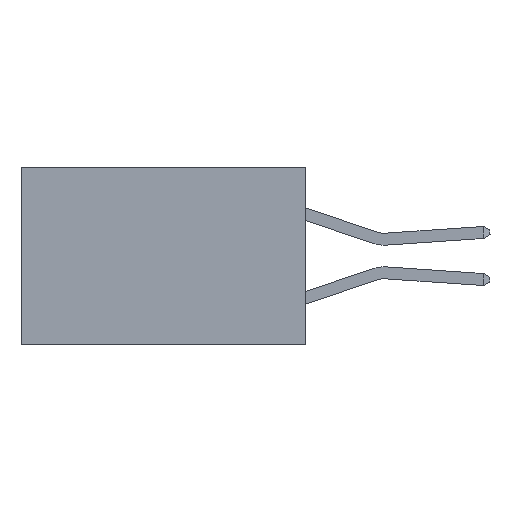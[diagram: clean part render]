
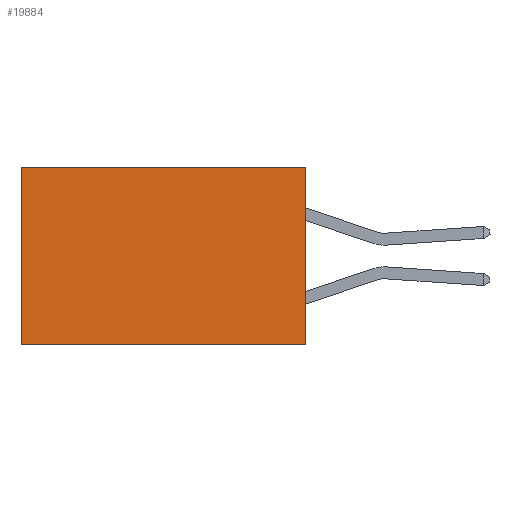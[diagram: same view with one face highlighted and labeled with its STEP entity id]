
A CAD part, left-side view. The second image highlights one B-rep face of the part: STEP entity #19884.
In plain terms, the highlighted planar face has unit normal (-1, 0, 0).
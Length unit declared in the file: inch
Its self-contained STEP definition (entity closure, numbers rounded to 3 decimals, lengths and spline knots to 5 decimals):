
#1234 = EDGE_CURVE ( 'NONE', #11306, #12728, #7090, .T. ) ;
#1339 = ORIENTED_EDGE ( 'NONE', *, *, #17410, .F. ) ;
#1686 = VECTOR ( 'NONE', #3702, 39.37008 ) ;
#2017 = DIRECTION ( 'NONE',  ( 0., 0., -1. ) ) ;
#2147 = AXIS2_PLACEMENT_3D ( 'NONE', #26123, #14279, #2017 ) ;
#3013 = CARTESIAN_POINT ( 'NONE',  ( 0.277, 0., 0. ) ) ;
#3610 = ORIENTED_EDGE ( 'NONE', *, *, #9936, .T. ) ;
#3702 = DIRECTION ( 'NONE',  ( 0., 1., 0. ) ) ;
#3708 = VERTEX_POINT ( 'NONE', #13649 ) ;
#4293 = ORIENTED_EDGE ( 'NONE', *, *, #5813, .F. ) ;
#5003 = EDGE_LOOP ( 'NONE', ( #3610, #4293, #1339, #12334 ) ) ;
#5049 = LINE ( 'NONE', #21857, #15259 ) ;
#5813 = EDGE_CURVE ( 'NONE', #3708, #24975, #5049, .T. ) ;
#6667 = LINE ( 'NONE', #12397, #22193 ) ;
#7090 = LINE ( 'NONE', #3013, #1686 ) ;
#7598 = CARTESIAN_POINT ( 'NONE',  ( 0.277, 0., -0.37 ) ) ;
#9936 = EDGE_CURVE ( 'NONE', #12728, #24975, #6667, .T. ) ;
#10819 = CARTESIAN_POINT ( 'NONE',  ( 0.277, 0.59, 0. ) ) ;
#11036 = VECTOR ( 'NONE', #11730, 39.37008 ) ;
#11306 = VERTEX_POINT ( 'NONE', #16877 ) ;
#11730 = DIRECTION ( 'NONE',  ( 0., 0., -1. ) ) ;
#12334 = ORIENTED_EDGE ( 'NONE', *, *, #1234, .T. ) ;
#12397 = CARTESIAN_POINT ( 'NONE',  ( 0.277, 0.59, -0.37 ) ) ;
#12728 = VERTEX_POINT ( 'NONE', #10819 ) ;
#13649 = CARTESIAN_POINT ( 'NONE',  ( 0.277, 0., -0.37 ) ) ;
#14279 = DIRECTION ( 'NONE',  ( 1., 0., 0. ) ) ;
#14931 = DIRECTION ( 'NONE',  ( 0., 1., 0. ) ) ;
#15259 = VECTOR ( 'NONE', #14931, 39.37008 ) ;
#16471 = LINE ( 'NONE', #7598, #11036 ) ;
#16877 = CARTESIAN_POINT ( 'NONE',  ( 0.277, 0., 0. ) ) ;
#16982 = CARTESIAN_POINT ( 'NONE',  ( 0.277, 0.59, -0.37 ) ) ;
#17410 = EDGE_CURVE ( 'NONE', #11306, #3708, #16471, .T. ) ;
#19884 = ADVANCED_FACE ( 'NONE', ( #25664 ), #25020, .F. ) ;
#21857 = CARTESIAN_POINT ( 'NONE',  ( 0.277, 0., -0.37 ) ) ;
#22193 = VECTOR ( 'NONE', #24401, 39.37008 ) ;
#24401 = DIRECTION ( 'NONE',  ( 0., 0., -1. ) ) ;
#24975 = VERTEX_POINT ( 'NONE', #16982 ) ;
#25020 = PLANE ( 'NONE',  #2147 ) ;
#25664 = FACE_OUTER_BOUND ( 'NONE', #5003, .T. ) ;
#26123 = CARTESIAN_POINT ( 'NONE',  ( 0.277, 0., -0.37 ) ) ;
